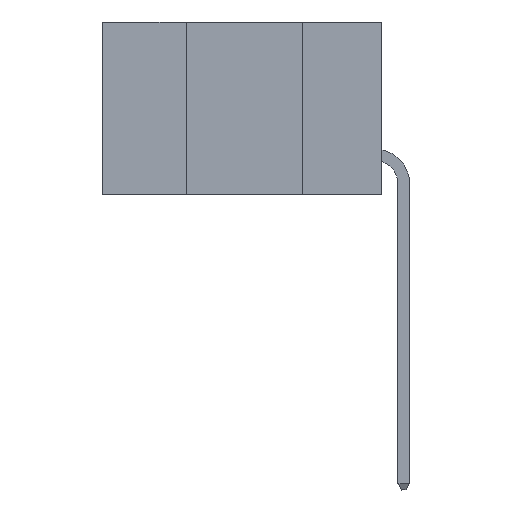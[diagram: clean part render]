
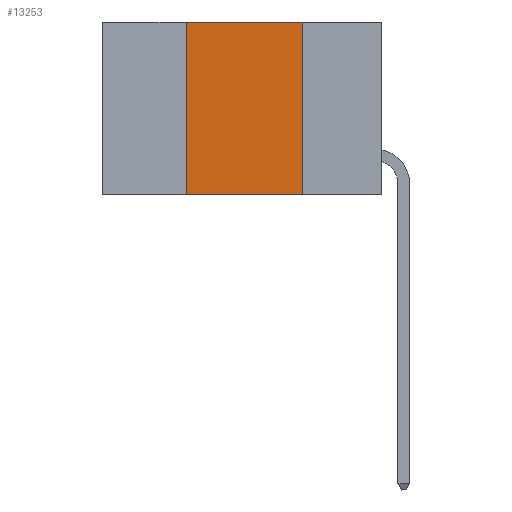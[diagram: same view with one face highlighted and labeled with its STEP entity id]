
A CAD part, left-side view. The second image highlights one B-rep face of the part: STEP entity #13253.
In plain terms, the highlighted planar face has unit normal (-1, 0, 0).
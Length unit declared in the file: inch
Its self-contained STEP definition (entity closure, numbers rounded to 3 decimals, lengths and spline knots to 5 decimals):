
#3017 = EDGE_CURVE ( 'NONE', #6850, #6056, #28260, .T. ) ;
#3104 = VERTEX_POINT ( 'NONE', #34098 ) ;
#3641 = EDGE_CURVE ( 'NONE', #6056, #17781, #25680, .T. ) ;
#4489 = DIRECTION ( 'NONE',  ( 0., 0., -1. ) ) ;
#4533 = CARTESIAN_POINT ( 'NONE',  ( 0., 0.6, 0. ) ) ;
#6056 = VERTEX_POINT ( 'NONE', #32892 ) ;
#6270 = LINE ( 'NONE', #27472, #18437 ) ;
#6850 = VERTEX_POINT ( 'NONE', #20552 ) ;
#9476 = CARTESIAN_POINT ( 'NONE',  ( 0., 0.17, -0.37 ) ) ;
#9614 = ORIENTED_EDGE ( 'NONE', *, *, #3017, .F. ) ;
#10849 = VECTOR ( 'NONE', #12889, 39.37008 ) ;
#10982 = DIRECTION ( 'NONE',  ( 0., -1., 0. ) ) ;
#12889 = DIRECTION ( 'NONE',  ( 0., -1., 0. ) ) ;
#13253 = ADVANCED_FACE ( 'NONE', ( #21964 ), #22741, .F. ) ;
#16735 = ORIENTED_EDGE ( 'NONE', *, *, #3641, .F. ) ;
#17283 = VECTOR ( 'NONE', #10982, 39.37008 ) ;
#17781 = VERTEX_POINT ( 'NONE', #9476 ) ;
#18437 = VECTOR ( 'NONE', #30002, 39.37008 ) ;
#19734 = EDGE_CURVE ( 'NONE', #3104, #17781, #25781, .T. ) ;
#20119 = CARTESIAN_POINT ( 'NONE',  ( 0., 0.6, -0.37 ) ) ;
#20552 = CARTESIAN_POINT ( 'NONE',  ( 0., 0.42, 0. ) ) ;
#21163 = ORIENTED_EDGE ( 'NONE', *, *, #24352, .F. ) ;
#21964 = FACE_OUTER_BOUND ( 'NONE', #36485, .T. ) ;
#22741 = PLANE ( 'NONE',  #37343 ) ;
#24352 = EDGE_CURVE ( 'NONE', #3104, #6850, #6270, .T. ) ;
#24899 = DIRECTION ( 'NONE',  ( 0., 0., -1. ) ) ;
#25486 = ORIENTED_EDGE ( 'NONE', *, *, #19734, .T. ) ;
#25680 = LINE ( 'NONE', #31130, #30768 ) ;
#25781 = LINE ( 'NONE', #20119, #17283 ) ;
#27472 = CARTESIAN_POINT ( 'NONE',  ( 0., 0.42, 0. ) ) ;
#28014 = DIRECTION ( 'NONE',  ( 1., 0., 0. ) ) ;
#28260 = LINE ( 'NONE', #4533, #10849 ) ;
#28398 = CARTESIAN_POINT ( 'NONE',  ( 0., 0.6, 0. ) ) ;
#30002 = DIRECTION ( 'NONE',  ( 0., 0., 1. ) ) ;
#30768 = VECTOR ( 'NONE', #4489, 39.37008 ) ;
#31130 = CARTESIAN_POINT ( 'NONE',  ( 0., 0.17, 0. ) ) ;
#32892 = CARTESIAN_POINT ( 'NONE',  ( 0., 0.17, 0. ) ) ;
#34098 = CARTESIAN_POINT ( 'NONE',  ( 0., 0.42, -0.37 ) ) ;
#36485 = EDGE_LOOP ( 'NONE', ( #16735, #9614, #21163, #25486 ) ) ;
#37343 = AXIS2_PLACEMENT_3D ( 'NONE', #28398, #28014, #24899 ) ;
